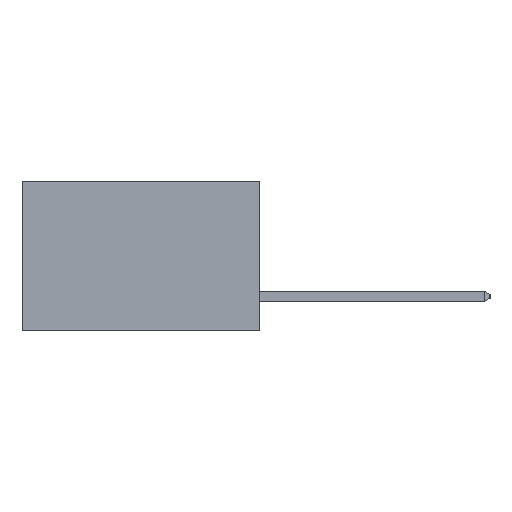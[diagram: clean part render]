
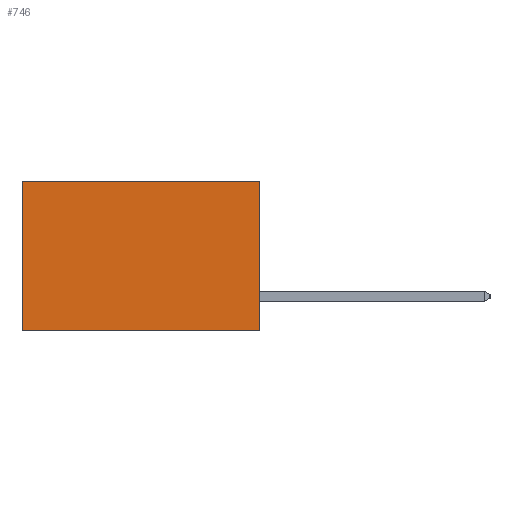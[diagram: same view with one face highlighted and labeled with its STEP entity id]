
A CAD part, left-side view. The second image highlights one B-rep face of the part: STEP entity #746.
In plain terms, the highlighted planar face has unit normal (-1, 0, 0).
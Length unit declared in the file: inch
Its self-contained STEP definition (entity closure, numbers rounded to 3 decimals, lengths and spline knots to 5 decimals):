
#468 = EDGE_CURVE ( 'NONE', #6033, #11491, #12866, .T. ) ;
#499 = ORIENTED_EDGE ( 'NONE', *, *, #468, .T. ) ;
#746 = ADVANCED_FACE ( 'NONE', ( #22011 ), #22463, .F. ) ;
#1714 = AXIS2_PLACEMENT_3D ( 'NONE', #9511, #6097, #23912 ) ;
#4497 = CARTESIAN_POINT ( 'NONE',  ( 0.277, 0., 0. ) ) ;
#5014 = VECTOR ( 'NONE', #17763, 39.37008 ) ;
#5311 = CARTESIAN_POINT ( 'NONE',  ( 0.277, 0.59, 0. ) ) ;
#5359 = CARTESIAN_POINT ( 'NONE',  ( 0.277, 0.59, -0.37 ) ) ;
#6033 = VERTEX_POINT ( 'NONE', #29716 ) ;
#6097 = DIRECTION ( 'NONE',  ( 1., 0., 0. ) ) ;
#9511 = CARTESIAN_POINT ( 'NONE',  ( 0.277, 0., -0.37 ) ) ;
#11491 = VERTEX_POINT ( 'NONE', #5311 ) ;
#11913 = DIRECTION ( 'NONE',  ( 0., 1., 0. ) ) ;
#12866 = LINE ( 'NONE', #4497, #32241 ) ;
#13009 = DIRECTION ( 'NONE',  ( 0., 0., -1. ) ) ;
#14192 = CARTESIAN_POINT ( 'NONE',  ( 0.277, 0., -0.37 ) ) ;
#15553 = LINE ( 'NONE', #5359, #20739 ) ;
#16430 = CARTESIAN_POINT ( 'NONE',  ( 0.277, 0.59, -0.37 ) ) ;
#16720 = DIRECTION ( 'NONE',  ( 0., 1., 0. ) ) ;
#16826 = EDGE_LOOP ( 'NONE', ( #27913, #29687, #25500, #499 ) ) ;
#17763 = DIRECTION ( 'NONE',  ( 0., 0., -1. ) ) ;
#17880 = VECTOR ( 'NONE', #16720, 39.37008 ) ;
#18797 = VERTEX_POINT ( 'NONE', #16430 ) ;
#18900 = VERTEX_POINT ( 'NONE', #24450 ) ;
#19408 = LINE ( 'NONE', #20207, #5014 ) ;
#20207 = CARTESIAN_POINT ( 'NONE',  ( 0.277, 0., -0.37 ) ) ;
#20446 = EDGE_CURVE ( 'NONE', #6033, #18900, #19408, .T. ) ;
#20739 = VECTOR ( 'NONE', #13009, 39.37008 ) ;
#22011 = FACE_OUTER_BOUND ( 'NONE', #16826, .T. ) ;
#22463 = PLANE ( 'NONE',  #1714 ) ;
#23912 = DIRECTION ( 'NONE',  ( 0., 0., -1. ) ) ;
#24450 = CARTESIAN_POINT ( 'NONE',  ( 0.277, 0., -0.37 ) ) ;
#24776 = EDGE_CURVE ( 'NONE', #11491, #18797, #15553, .T. ) ;
#25500 = ORIENTED_EDGE ( 'NONE', *, *, #20446, .F. ) ;
#27913 = ORIENTED_EDGE ( 'NONE', *, *, #24776, .T. ) ;
#29687 = ORIENTED_EDGE ( 'NONE', *, *, #29970, .F. ) ;
#29716 = CARTESIAN_POINT ( 'NONE',  ( 0.277, 0., 0. ) ) ;
#29970 = EDGE_CURVE ( 'NONE', #18900, #18797, #31302, .T. ) ;
#31302 = LINE ( 'NONE', #14192, #17880 ) ;
#32241 = VECTOR ( 'NONE', #11913, 39.37008 ) ;
